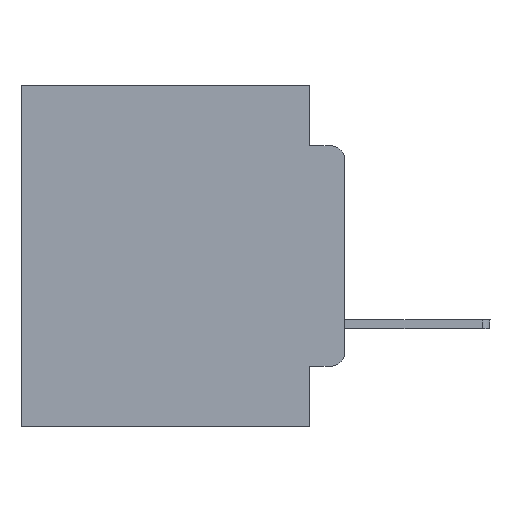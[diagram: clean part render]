
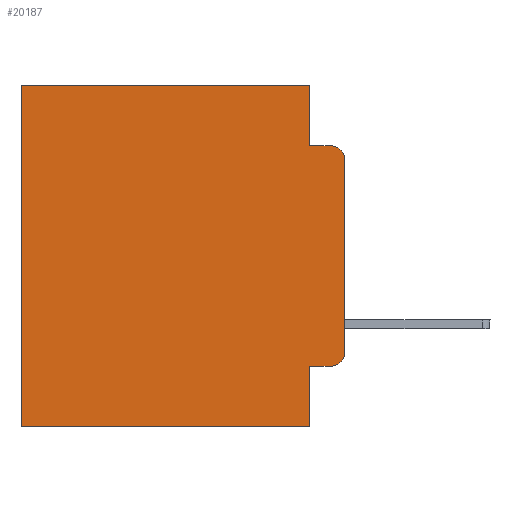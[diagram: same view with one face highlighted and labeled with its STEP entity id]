
A CAD part, left-side view. The second image highlights one B-rep face of the part: STEP entity #20187.
In plain terms, the highlighted planar face has unit normal (-1, 0, 0).
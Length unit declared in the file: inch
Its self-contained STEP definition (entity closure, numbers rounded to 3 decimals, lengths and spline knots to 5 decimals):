
#93 = EDGE_CURVE ( 'NONE', #20357, #9292, #3522, .T. ) ;
#596 = CIRCLE ( 'NONE', #16186, 0.02 ) ;
#970 = EDGE_CURVE ( 'NONE', #8468, #22360, #22666, .T. ) ;
#1117 = CARTESIAN_POINT ( 'NONE',  ( 0.298, 0.051, -0.5 ) ) ;
#1294 = EDGE_CURVE ( 'NONE', #1492, #21844, #15507, .T. ) ;
#1341 = ORIENTED_EDGE ( 'NONE', *, *, #10507, .T. ) ;
#1461 = VERTEX_POINT ( 'NONE', #8307 ) ;
#1492 = VERTEX_POINT ( 'NONE', #19509 ) ;
#3101 = VERTEX_POINT ( 'NONE', #1117 ) ;
#3522 = CIRCLE ( 'NONE', #14201, 0.02 ) ;
#3559 = VECTOR ( 'NONE', #16080, 39.37008 ) ;
#3730 = DIRECTION ( 'NONE',  ( 0., -1., 0. ) ) ;
#3966 = EDGE_CURVE ( 'NONE', #8468, #1492, #25089, .T. ) ;
#4418 = LINE ( 'NONE', #25375, #24557 ) ;
#5537 = DIRECTION ( 'NONE',  ( -1., 0., 0. ) ) ;
#6237 = CARTESIAN_POINT ( 'NONE',  ( 0.298, 0., -0.1085 ) ) ;
#6657 = DIRECTION ( 'NONE',  ( 0., -1., 0. ) ) ;
#6952 = ORIENTED_EDGE ( 'NONE', *, *, #21649, .T. ) ;
#7112 = DIRECTION ( 'NONE',  ( -1., 0., 0. ) ) ;
#7323 = ORIENTED_EDGE ( 'NONE', *, *, #24474, .F. ) ;
#7739 = LINE ( 'NONE', #27047, #16261 ) ;
#7769 = DIRECTION ( 'NONE',  ( 0., 0., -1. ) ) ;
#7879 = DIRECTION ( 'NONE',  ( 0., 0., -1. ) ) ;
#8166 = CARTESIAN_POINT ( 'NONE',  ( 0.298, 0., 0. ) ) ;
#8307 = CARTESIAN_POINT ( 'NONE',  ( 0.298, 0.051, -0.4115 ) ) ;
#8401 = ORIENTED_EDGE ( 'NONE', *, *, #3966, .F. ) ;
#8449 = DIRECTION ( 'NONE',  ( 0., 1., 0. ) ) ;
#8468 = VERTEX_POINT ( 'NONE', #12190 ) ;
#9062 = CARTESIAN_POINT ( 'NONE',  ( 0.298, 0.02, -0.1085 ) ) ;
#9063 = CARTESIAN_POINT ( 'NONE',  ( 0.298, 0.051, -0.0885 ) ) ;
#9292 = VERTEX_POINT ( 'NONE', #14198 ) ;
#9511 = CARTESIAN_POINT ( 'NONE',  ( 0.298, 0., 0. ) ) ;
#9994 = FACE_OUTER_BOUND ( 'NONE', #16802, .T. ) ;
#10267 = CARTESIAN_POINT ( 'NONE',  ( 0.298, 0.051, 0. ) ) ;
#10507 = EDGE_CURVE ( 'NONE', #25491, #21844, #596, .T. ) ;
#10686 = LINE ( 'NONE', #23153, #26841 ) ;
#11953 = CARTESIAN_POINT ( 'NONE',  ( 0.298, 0.02, -0.3915 ) ) ;
#12190 = CARTESIAN_POINT ( 'NONE',  ( 0.298, 0.051, 0. ) ) ;
#12976 = CARTESIAN_POINT ( 'NONE',  ( 0.298, 0.473, 0. ) ) ;
#13759 = AXIS2_PLACEMENT_3D ( 'NONE', #8166, #27208, #7769 ) ;
#14000 = DIRECTION ( 'NONE',  ( 0., 0., -1. ) ) ;
#14197 = DIRECTION ( 'NONE',  ( 0., 0., -1. ) ) ;
#14198 = CARTESIAN_POINT ( 'NONE',  ( 0.298, 0., -0.3915 ) ) ;
#14201 = AXIS2_PLACEMENT_3D ( 'NONE', #11953, #5537, #20915 ) ;
#14449 = CARTESIAN_POINT ( 'NONE',  ( 0.298, 0.02, -0.0885 ) ) ;
#14658 = EDGE_CURVE ( 'NONE', #25491, #9292, #7739, .T. ) ;
#15045 = ORIENTED_EDGE ( 'NONE', *, *, #14658, .F. ) ;
#15173 = VECTOR ( 'NONE', #3730, 39.37008 ) ;
#15507 = LINE ( 'NONE', #9063, #15173 ) ;
#16080 = DIRECTION ( 'NONE',  ( 0., 1., 0. ) ) ;
#16186 = AXIS2_PLACEMENT_3D ( 'NONE', #9062, #7112, #24448 ) ;
#16261 = VECTOR ( 'NONE', #7879, 39.37008 ) ;
#16802 = EDGE_LOOP ( 'NONE', ( #15045, #1341, #17680, #8401, #25936, #26491, #22446, #7323, #6952, #25699 ) ) ;
#17115 = CARTESIAN_POINT ( 'NONE',  ( 0.298, 0.02, -0.4115 ) ) ;
#17583 = LINE ( 'NONE', #12976, #22253 ) ;
#17680 = ORIENTED_EDGE ( 'NONE', *, *, #1294, .F. ) ;
#17972 = EDGE_CURVE ( 'NONE', #22360, #18475, #17583, .T. ) ;
#18202 = CARTESIAN_POINT ( 'NONE',  ( 0.298, 0.051, 0. ) ) ;
#18475 = VERTEX_POINT ( 'NONE', #26352 ) ;
#19509 = CARTESIAN_POINT ( 'NONE',  ( 0.298, 0.051, -0.0885 ) ) ;
#20187 = ADVANCED_FACE ( 'NONE', ( #9994 ), #26934, .F. ) ;
#20357 = VERTEX_POINT ( 'NONE', #17115 ) ;
#20614 = VECTOR ( 'NONE', #14000, 39.37008 ) ;
#20915 = DIRECTION ( 'NONE',  ( 0., 0., -1. ) ) ;
#21287 = VECTOR ( 'NONE', #14197, 39.37008 ) ;
#21649 = EDGE_CURVE ( 'NONE', #1461, #20357, #4418, .T. ) ;
#21844 = VERTEX_POINT ( 'NONE', #14449 ) ;
#22253 = VECTOR ( 'NONE', #25973, 39.37008 ) ;
#22360 = VERTEX_POINT ( 'NONE', #22951 ) ;
#22446 = ORIENTED_EDGE ( 'NONE', *, *, #24279, .F. ) ;
#22666 = LINE ( 'NONE', #9511, #3559 ) ;
#22951 = CARTESIAN_POINT ( 'NONE',  ( 0.298, 0.473, 0. ) ) ;
#23153 = CARTESIAN_POINT ( 'NONE',  ( 0.298, 0., -0.5 ) ) ;
#24279 = EDGE_CURVE ( 'NONE', #3101, #18475, #10686, .T. ) ;
#24448 = DIRECTION ( 'NONE',  ( 0., 0., -1. ) ) ;
#24474 = EDGE_CURVE ( 'NONE', #1461, #3101, #26441, .T. ) ;
#24557 = VECTOR ( 'NONE', #6657, 39.37008 ) ;
#25089 = LINE ( 'NONE', #10267, #21287 ) ;
#25375 = CARTESIAN_POINT ( 'NONE',  ( 0.298, 0.051, -0.4115 ) ) ;
#25491 = VERTEX_POINT ( 'NONE', #6237 ) ;
#25699 = ORIENTED_EDGE ( 'NONE', *, *, #93, .T. ) ;
#25936 = ORIENTED_EDGE ( 'NONE', *, *, #970, .T. ) ;
#25973 = DIRECTION ( 'NONE',  ( 0., 0., -1. ) ) ;
#26352 = CARTESIAN_POINT ( 'NONE',  ( 0.298, 0.473, -0.5 ) ) ;
#26441 = LINE ( 'NONE', #18202, #20614 ) ;
#26491 = ORIENTED_EDGE ( 'NONE', *, *, #17972, .T. ) ;
#26841 = VECTOR ( 'NONE', #8449, 39.37008 ) ;
#26934 = PLANE ( 'NONE',  #13759 ) ;
#27047 = CARTESIAN_POINT ( 'NONE',  ( 0.298, 0., 0. ) ) ;
#27208 = DIRECTION ( 'NONE',  ( 1., 0., 0. ) ) ;
